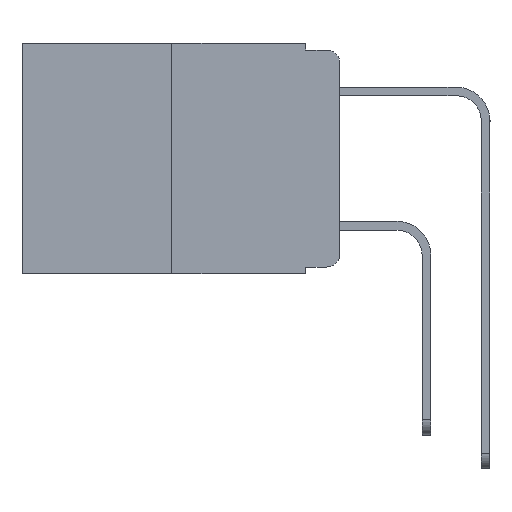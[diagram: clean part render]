
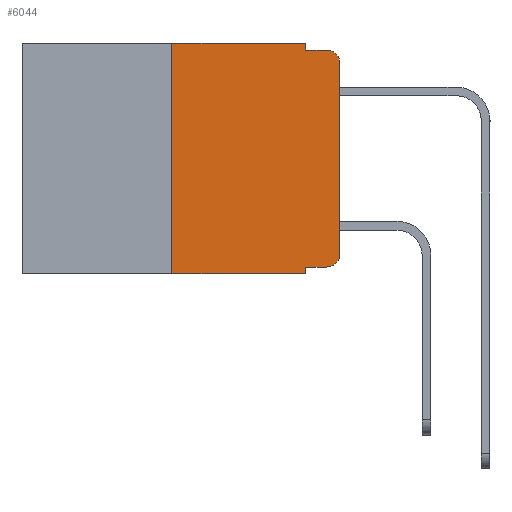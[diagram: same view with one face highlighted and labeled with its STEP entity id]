
A CAD part, left-side view. The second image highlights one B-rep face of the part: STEP entity #6044.
In plain terms, the highlighted planar face has unit normal (-1, 0, 0).
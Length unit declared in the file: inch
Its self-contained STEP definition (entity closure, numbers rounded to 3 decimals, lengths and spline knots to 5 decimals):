
#54 = EDGE_CURVE ( 'NONE', #4182, #925, #4015, .T. ) ;
#208 = LINE ( 'NONE', #10933, #8384 ) ;
#399 = EDGE_CURVE ( 'NONE', #8723, #10164, #15129, .T. ) ;
#481 = DIRECTION ( 'NONE',  ( 0., 0., -1. ) ) ;
#925 = VERTEX_POINT ( 'NONE', #3002 ) ;
#1172 = EDGE_CURVE ( 'NONE', #17404, #4182, #15758, .T. ) ;
#1425 = CARTESIAN_POINT ( 'NONE',  ( 0., 0.25, 0. ) ) ;
#2256 = CARTESIAN_POINT ( 'NONE',  ( 0., 0.02, -0.03 ) ) ;
#2285 = DIRECTION ( 'NONE',  ( -1., 0., 0. ) ) ;
#2360 = VERTEX_POINT ( 'NONE', #5767 ) ;
#2520 = CARTESIAN_POINT ( 'NONE',  ( 0., 0.473, -0.343 ) ) ;
#2886 = VECTOR ( 'NONE', #17066, 39.37008 ) ;
#2905 = CARTESIAN_POINT ( 'NONE',  ( 0., 0.473, 0. ) ) ;
#3002 = CARTESIAN_POINT ( 'NONE',  ( 0., 0.02, -0.01 ) ) ;
#3256 = CARTESIAN_POINT ( 'NONE',  ( 0., 0., -0.313 ) ) ;
#3831 = LINE ( 'NONE', #1425, #11982 ) ;
#3991 = ORIENTED_EDGE ( 'NONE', *, *, #399, .F. ) ;
#4008 = CARTESIAN_POINT ( 'NONE',  ( 0., 0.051, -0.01 ) ) ;
#4015 = CIRCLE ( 'NONE', #14650, 0.02 ) ;
#4034 = ORIENTED_EDGE ( 'NONE', *, *, #14619, .F. ) ;
#4153 = DIRECTION ( 'NONE',  ( 0., -1., 0. ) ) ;
#4182 = VERTEX_POINT ( 'NONE', #18733 ) ;
#4591 = DIRECTION ( 'NONE',  ( 0., 0., -1. ) ) ;
#4623 = EDGE_CURVE ( 'NONE', #2360, #8898, #8313, .T. ) ;
#5626 = CARTESIAN_POINT ( 'NONE',  ( 0., 0.051, -0.343 ) ) ;
#5648 = ORIENTED_EDGE ( 'NONE', *, *, #1172, .T. ) ;
#5767 = CARTESIAN_POINT ( 'NONE',  ( 0., 0.25, -0.343 ) ) ;
#6044 = ADVANCED_FACE ( 'NONE', ( #7246 ), #6168, .F. ) ;
#6168 = PLANE ( 'NONE',  #15251 ) ;
#6950 = VECTOR ( 'NONE', #10077, 39.37008 ) ;
#6967 = CIRCLE ( 'NONE', #10491, 0.02 ) ;
#6989 = CARTESIAN_POINT ( 'NONE',  ( 0., 0.051, -0.333 ) ) ;
#7077 = VECTOR ( 'NONE', #15352, 39.37008 ) ;
#7246 = FACE_OUTER_BOUND ( 'NONE', #16238, .T. ) ;
#7493 = LINE ( 'NONE', #6989, #15034 ) ;
#7724 = ORIENTED_EDGE ( 'NONE', *, *, #54, .T. ) ;
#8080 = LINE ( 'NONE', #19316, #16092 ) ;
#8258 = CARTESIAN_POINT ( 'NONE',  ( 0., 0.473, 0. ) ) ;
#8313 = LINE ( 'NONE', #2520, #15836 ) ;
#8384 = VECTOR ( 'NONE', #12572, 39.37008 ) ;
#8502 = CARTESIAN_POINT ( 'NONE',  ( 0., 0.25, 0. ) ) ;
#8723 = VERTEX_POINT ( 'NONE', #8502 ) ;
#8898 = VERTEX_POINT ( 'NONE', #5626 ) ;
#8979 = CARTESIAN_POINT ( 'NONE',  ( 0., 0.02, -0.313 ) ) ;
#9448 = CARTESIAN_POINT ( 'NONE',  ( 0., 0.051, -0.333 ) ) ;
#9700 = DIRECTION ( 'NONE',  ( 0., -1., 0. ) ) ;
#10077 = DIRECTION ( 'NONE',  ( 0., 0., -1. ) ) ;
#10164 = VERTEX_POINT ( 'NONE', #15264 ) ;
#10491 = AXIS2_PLACEMENT_3D ( 'NONE', #8979, #20031, #10598 ) ;
#10518 = ORIENTED_EDGE ( 'NONE', *, *, #16697, .F. ) ;
#10562 = VERTEX_POINT ( 'NONE', #13320 ) ;
#10598 = DIRECTION ( 'NONE',  ( 0., 0., -1. ) ) ;
#10625 = ORIENTED_EDGE ( 'NONE', *, *, #4623, .T. ) ;
#10774 = ORIENTED_EDGE ( 'NONE', *, *, #19820, .F. ) ;
#10933 = CARTESIAN_POINT ( 'NONE',  ( 0., 0.051, 0. ) ) ;
#11266 = LINE ( 'NONE', #13271, #6950 ) ;
#11393 = EDGE_CURVE ( 'NONE', #10562, #17404, #6967, .T. ) ;
#11982 = VECTOR ( 'NONE', #20578, 39.37008 ) ;
#12572 = DIRECTION ( 'NONE',  ( 0., 0., -1. ) ) ;
#13271 = CARTESIAN_POINT ( 'NONE',  ( 0., 0.051, 0. ) ) ;
#13320 = CARTESIAN_POINT ( 'NONE',  ( 0., 0.02, -0.333 ) ) ;
#13569 = EDGE_CURVE ( 'NONE', #17801, #10562, #7493, .T. ) ;
#14319 = DIRECTION ( 'NONE',  ( 1., 0., 0. ) ) ;
#14619 = EDGE_CURVE ( 'NONE', #17801, #8898, #11266, .T. ) ;
#14650 = AXIS2_PLACEMENT_3D ( 'NONE', #2256, #2285, #481 ) ;
#14680 = ORIENTED_EDGE ( 'NONE', *, *, #13569, .T. ) ;
#15034 = VECTOR ( 'NONE', #18154, 39.37008 ) ;
#15129 = LINE ( 'NONE', #8258, #7077 ) ;
#15251 = AXIS2_PLACEMENT_3D ( 'NONE', #2905, #14319, #4591 ) ;
#15264 = CARTESIAN_POINT ( 'NONE',  ( 0., 0.051, 0. ) ) ;
#15352 = DIRECTION ( 'NONE',  ( 0., -1., 0. ) ) ;
#15671 = EDGE_CURVE ( 'NONE', #2360, #8723, #3831, .T. ) ;
#15758 = LINE ( 'NONE', #17119, #2886 ) ;
#15836 = VECTOR ( 'NONE', #4153, 39.37008 ) ;
#16092 = VECTOR ( 'NONE', #9700, 39.37008 ) ;
#16144 = ORIENTED_EDGE ( 'NONE', *, *, #11393, .T. ) ;
#16238 = EDGE_LOOP ( 'NONE', ( #5648, #7724, #10774, #10518, #3991, #17084, #10625, #4034, #14680, #16144 ) ) ;
#16697 = EDGE_CURVE ( 'NONE', #10164, #17177, #208, .T. ) ;
#17066 = DIRECTION ( 'NONE',  ( 0., 0., 1. ) ) ;
#17084 = ORIENTED_EDGE ( 'NONE', *, *, #15671, .F. ) ;
#17119 = CARTESIAN_POINT ( 'NONE',  ( 0., 0., 0. ) ) ;
#17177 = VERTEX_POINT ( 'NONE', #4008 ) ;
#17404 = VERTEX_POINT ( 'NONE', #3256 ) ;
#17801 = VERTEX_POINT ( 'NONE', #9448 ) ;
#18154 = DIRECTION ( 'NONE',  ( 0., -1., 0. ) ) ;
#18733 = CARTESIAN_POINT ( 'NONE',  ( 0., 0., -0.03 ) ) ;
#19316 = CARTESIAN_POINT ( 'NONE',  ( 0., 0.051, -0.01 ) ) ;
#19820 = EDGE_CURVE ( 'NONE', #17177, #925, #8080, .T. ) ;
#20031 = DIRECTION ( 'NONE',  ( -1., 0., 0. ) ) ;
#20578 = DIRECTION ( 'NONE',  ( 0., 0., 1. ) ) ;
